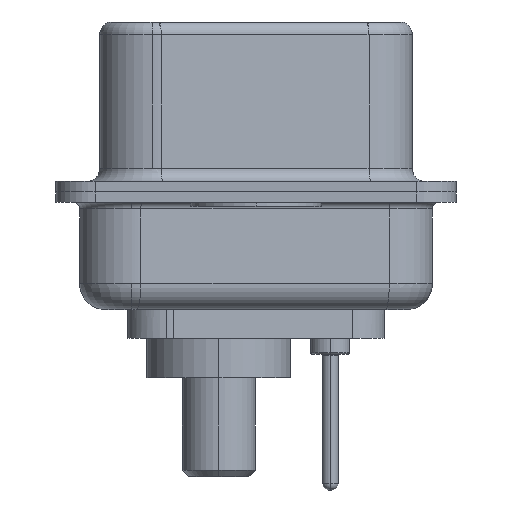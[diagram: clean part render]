
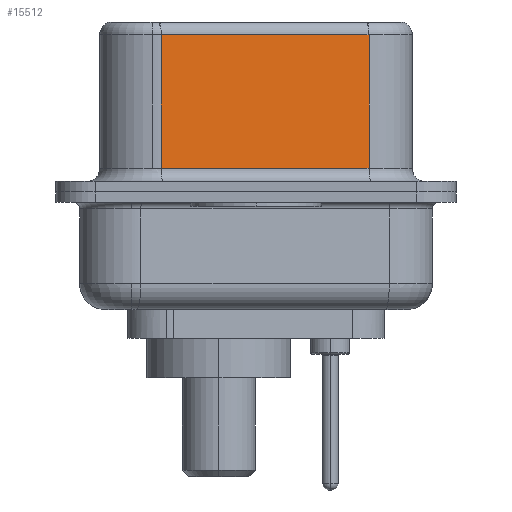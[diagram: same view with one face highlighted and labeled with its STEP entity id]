
A CAD part, left-side view. The second image highlights one B-rep face of the part: STEP entity #15512.
In plain terms, the highlighted planar face has unit normal (-0.985, -0.174, 0).
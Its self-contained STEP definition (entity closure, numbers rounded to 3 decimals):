
#1014 = EDGE_LOOP ( 'NONE', ( #18843, #15731, #15713, #9127 ) ) ;
#1451 = DIRECTION ( 'NONE',  ( 0., 0., -1. ) ) ;
#1638 = EDGE_CURVE ( 'NONE', #18327, #5674, #6390, .T. ) ;
#2261 = CARTESIAN_POINT ( 'NONE',  ( 5.132, -4.322, 6.02 ) ) ;
#2433 = VECTOR ( 'NONE', #1451, 1000. ) ;
#4074 = CARTESIAN_POINT ( 'NONE',  ( 5.132, -4.322, 0.9 ) ) ;
#5519 = VERTEX_POINT ( 'NONE', #18884 ) ;
#5674 = VERTEX_POINT ( 'NONE', #4074 ) ;
#6390 = LINE ( 'NONE', #15375, #10574 ) ;
#7124 = FACE_OUTER_BOUND ( 'NONE', #1014, .T. ) ;
#7390 = CARTESIAN_POINT ( 'NONE',  ( 5.132, -4.322, 6.52 ) ) ;
#8108 = CARTESIAN_POINT ( 'NONE',  ( 3.73, 3.628, 6.02 ) ) ;
#8177 = EDGE_CURVE ( 'NONE', #14326, #18327, #17533, .T. ) ;
#9127 = ORIENTED_EDGE ( 'NONE', *, *, #1638, .T. ) ;
#9507 = PLANE ( 'NONE',  #11254 ) ;
#9778 = CARTESIAN_POINT ( 'NONE',  ( 3.73, 3.628, 0.9 ) ) ;
#10574 = VECTOR ( 'NONE', #12450, 1000. ) ;
#10881 = LINE ( 'NONE', #7390, #2433 ) ;
#11119 = DIRECTION ( 'NONE',  ( 0.985, 0.174, 0. ) ) ;
#11254 = AXIS2_PLACEMENT_3D ( 'NONE', #17181, #11119, #17043 ) ;
#11442 = DIRECTION ( 'NONE',  ( -0.174, 0.985, 0. ) ) ;
#11865 = DIRECTION ( 'NONE',  ( 0., 0., -1. ) ) ;
#12450 = DIRECTION ( 'NONE',  ( 0.174, -0.985, 0. ) ) ;
#13400 = CARTESIAN_POINT ( 'NONE',  ( 3.73, 3.628, 6.52 ) ) ;
#14326 = VERTEX_POINT ( 'NONE', #8108 ) ;
#14613 = EDGE_CURVE ( 'NONE', #5519, #5674, #10881, .T. ) ;
#14733 = LINE ( 'NONE', #2261, #18208 ) ;
#15375 = CARTESIAN_POINT ( 'NONE',  ( 5.132, -4.322, 0.9 ) ) ;
#15512 = ADVANCED_FACE ( 'NONE', ( #7124 ), #9507, .F. ) ;
#15713 = ORIENTED_EDGE ( 'NONE', *, *, #8177, .T. ) ;
#15731 = ORIENTED_EDGE ( 'NONE', *, *, #17334, .T. ) ;
#17043 = DIRECTION ( 'NONE',  ( -0.174, 0.985, 0. ) ) ;
#17078 = VECTOR ( 'NONE', #11865, 1000. ) ;
#17181 = CARTESIAN_POINT ( 'NONE',  ( 5.132, -4.322, 6.52 ) ) ;
#17334 = EDGE_CURVE ( 'NONE', #5519, #14326, #14733, .T. ) ;
#17533 = LINE ( 'NONE', #13400, #17078 ) ;
#18208 = VECTOR ( 'NONE', #11442, 1000. ) ;
#18327 = VERTEX_POINT ( 'NONE', #9778 ) ;
#18843 = ORIENTED_EDGE ( 'NONE', *, *, #14613, .F. ) ;
#18884 = CARTESIAN_POINT ( 'NONE',  ( 5.132, -4.322, 6.02 ) ) ;
